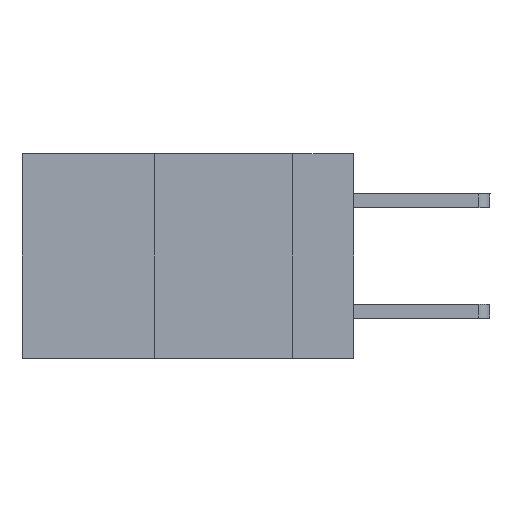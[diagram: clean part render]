
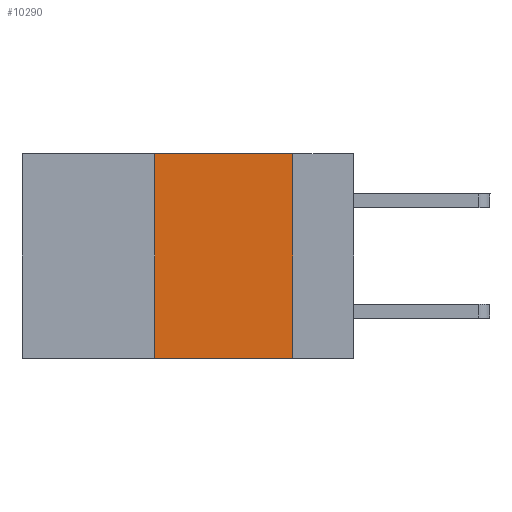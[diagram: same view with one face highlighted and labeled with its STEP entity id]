
A CAD part, left-side view. The second image highlights one B-rep face of the part: STEP entity #10290.
In plain terms, the highlighted planar face has unit normal (-1, 0, 0).
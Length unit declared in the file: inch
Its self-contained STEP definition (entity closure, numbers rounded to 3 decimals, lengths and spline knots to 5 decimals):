
#564 = ORIENTED_EDGE ( 'NONE', *, *, #5065, .F. ) ;
#707 = EDGE_LOOP ( 'NONE', ( #9672, #4405, #564, #10476 ) ) ;
#962 = LINE ( 'NONE', #5039, #3465 ) ;
#1638 = AXIS2_PLACEMENT_3D ( 'NONE', #2277, #6044, #11247 ) ;
#1685 = CARTESIAN_POINT ( 'NONE',  ( 0., 0.6, -0.37 ) ) ;
#2277 = CARTESIAN_POINT ( 'NONE',  ( 0., 0.6, 0. ) ) ;
#3196 = FACE_OUTER_BOUND ( 'NONE', #707, .T. ) ;
#3465 = VECTOR ( 'NONE', #6018, 39.37008 ) ;
#3745 = CARTESIAN_POINT ( 'NONE',  ( 0., 0.11, 0. ) ) ;
#3881 = EDGE_CURVE ( 'NONE', #5413, #5102, #962, .T. ) ;
#4105 = CARTESIAN_POINT ( 'NONE',  ( 0., 0.36, 0. ) ) ;
#4252 = CARTESIAN_POINT ( 'NONE',  ( 0., 0.36, 0. ) ) ;
#4405 = ORIENTED_EDGE ( 'NONE', *, *, #3881, .F. ) ;
#5039 = CARTESIAN_POINT ( 'NONE',  ( 0., 0.6, 0. ) ) ;
#5065 = EDGE_CURVE ( 'NONE', #10132, #5413, #11734, .T. ) ;
#5102 = VERTEX_POINT ( 'NONE', #7543 ) ;
#5217 = LINE ( 'NONE', #1685, #9741 ) ;
#5413 = VERTEX_POINT ( 'NONE', #4105 ) ;
#5613 = LINE ( 'NONE', #3745, #10916 ) ;
#5665 = CARTESIAN_POINT ( 'NONE',  ( 0., 0.11, -0.37 ) ) ;
#5725 = DIRECTION ( 'NONE',  ( 0., 0., -1. ) ) ;
#6018 = DIRECTION ( 'NONE',  ( 0., -1., 0. ) ) ;
#6044 = DIRECTION ( 'NONE',  ( 1., 0., 0. ) ) ;
#6340 = DIRECTION ( 'NONE',  ( 0., -1., 0. ) ) ;
#6395 = EDGE_CURVE ( 'NONE', #10132, #8713, #5217, .T. ) ;
#7042 = DIRECTION ( 'NONE',  ( 0., 0., 1. ) ) ;
#7076 = EDGE_CURVE ( 'NONE', #5102, #8713, #5613, .T. ) ;
#7543 = CARTESIAN_POINT ( 'NONE',  ( 0., 0.11, 0. ) ) ;
#7667 = CARTESIAN_POINT ( 'NONE',  ( 0., 0.36, -0.37 ) ) ;
#8713 = VERTEX_POINT ( 'NONE', #5665 ) ;
#9655 = VECTOR ( 'NONE', #7042, 39.37008 ) ;
#9672 = ORIENTED_EDGE ( 'NONE', *, *, #7076, .F. ) ;
#9741 = VECTOR ( 'NONE', #6340, 39.37008 ) ;
#10132 = VERTEX_POINT ( 'NONE', #7667 ) ;
#10290 = ADVANCED_FACE ( 'NONE', ( #3196 ), #10781, .F. ) ;
#10476 = ORIENTED_EDGE ( 'NONE', *, *, #6395, .T. ) ;
#10781 = PLANE ( 'NONE',  #1638 ) ;
#10916 = VECTOR ( 'NONE', #5725, 39.37008 ) ;
#11247 = DIRECTION ( 'NONE',  ( 0., 0., -1. ) ) ;
#11734 = LINE ( 'NONE', #4252, #9655 ) ;
